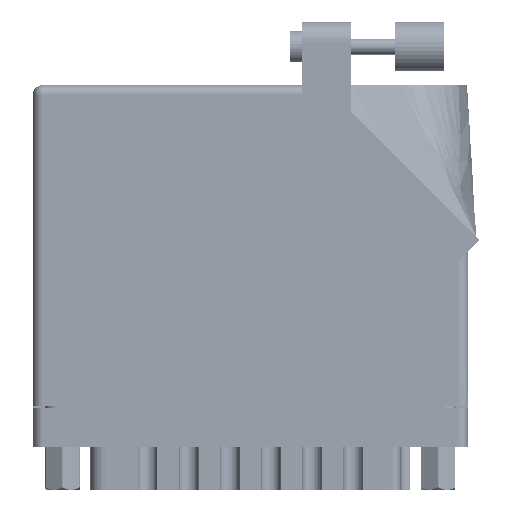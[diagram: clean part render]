
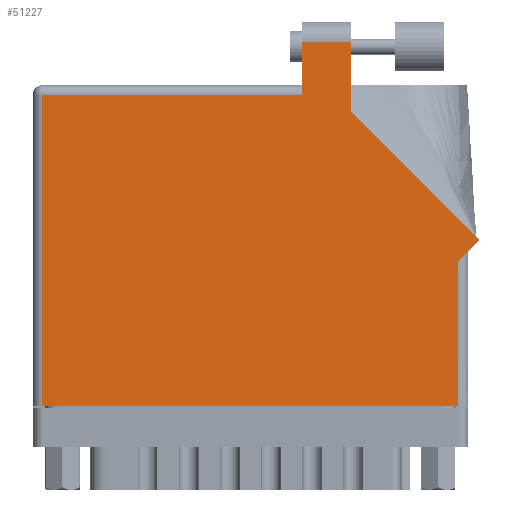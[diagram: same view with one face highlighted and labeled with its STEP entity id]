
A CAD part, front view. The second image highlights one B-rep face of the part: STEP entity #51227.
In plain terms, the highlighted face is planar.
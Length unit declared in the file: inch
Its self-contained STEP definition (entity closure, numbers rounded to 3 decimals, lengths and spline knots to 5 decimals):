
#69 = EDGE_CURVE ( 'NONE', #58738, #90624, #96330, .T. ) ;
#120 = VERTEX_POINT ( 'NONE', #54953 ) ;
#1323 = ORIENTED_EDGE ( 'NONE', *, *, #90444, .T. ) ;
#2523 = CARTESIAN_POINT ( 'NONE',  ( 0.062, 0., 0. ) ) ;
#3056 = ORIENTED_EDGE ( 'NONE', *, *, #69, .T. ) ;
#7707 = CARTESIAN_POINT ( 'NONE',  ( 2.755, 0.98, 0. ) ) ;
#7868 = DIRECTION ( 'NONE',  ( -0.707, 0.707, 0. ) ) ;
#9146 = LINE ( 'NONE', #7707, #66807 ) ;
#12510 = DIRECTION ( 'NONE',  ( 0., 0., -1. ) ) ;
#13361 = VECTOR ( 'NONE', #80149, 39.37008 ) ;
#14451 = CARTESIAN_POINT ( 'NONE',  ( 1.705, 1.968, 0. ) ) ;
#14509 = CARTESIAN_POINT ( 'NONE',  ( 0., 1.968, 0. ) ) ;
#16419 = LINE ( 'NONE', #42456, #101014 ) ;
#16767 = VECTOR ( 'NONE', #7868, 39.37008 ) ;
#20157 = LINE ( 'NONE', #26594, #27885 ) ;
#26452 = VERTEX_POINT ( 'NONE', #14451 ) ;
#26594 = CARTESIAN_POINT ( 'NONE',  ( 0.062, 0., 0. ) ) ;
#27885 = VECTOR ( 'NONE', #75751, 39.37008 ) ;
#28633 = LINE ( 'NONE', #75837, #69703 ) ;
#28959 = PLANE ( 'NONE',  #84256 ) ;
#30396 = EDGE_CURVE ( 'NONE', #26452, #61078, #36361, .T. ) ;
#31133 = CARTESIAN_POINT ( 'NONE',  ( 1.705, 2.305, 0. ) ) ;
#31562 = LINE ( 'NONE', #98910, #35449 ) ;
#32797 = CARTESIAN_POINT ( 'NONE',  ( 0.062, 1.968, 0. ) ) ;
#33068 = CARTESIAN_POINT ( 'NONE',  ( 1.705, 2.305, 0. ) ) ;
#35449 = VECTOR ( 'NONE', #82160, 39.37008 ) ;
#35515 = ORIENTED_EDGE ( 'NONE', *, *, #80331, .T. ) ;
#35644 = DIRECTION ( 'NONE',  ( 0., 1., 0. ) ) ;
#36361 = LINE ( 'NONE', #14509, #13361 ) ;
#36770 = VERTEX_POINT ( 'NONE', #53241 ) ;
#42456 = CARTESIAN_POINT ( 'NONE',  ( 2.012, 1.86442, 0. ) ) ;
#42857 = ORIENTED_EDGE ( 'NONE', *, *, #71810, .T. ) ;
#44968 = EDGE_CURVE ( 'NONE', #70366, #120, #48867, .T. ) ;
#48357 = ORIENTED_EDGE ( 'NONE', *, *, #69856, .T. ) ;
#48867 = LINE ( 'NONE', #105959, #16767 ) ;
#49530 = ORIENTED_EDGE ( 'NONE', *, *, #83313, .T. ) ;
#51227 = ADVANCED_FACE ( 'NONE', ( #67690 ), #28959, .F. ) ;
#53241 = CARTESIAN_POINT ( 'NONE',  ( 2.693, 0.918, 0. ) ) ;
#54953 = CARTESIAN_POINT ( 'NONE',  ( 2.012, 1.86442, 0. ) ) ;
#57809 = DIRECTION ( 'NONE',  ( 0.707, 0.707, 0. ) ) ;
#58738 = VERTEX_POINT ( 'NONE', #2523 ) ;
#61078 = VERTEX_POINT ( 'NONE', #32797 ) ;
#61192 = CARTESIAN_POINT ( 'NONE',  ( 0., 2.03, 0. ) ) ;
#61625 = EDGE_LOOP ( 'NONE', ( #1323, #42857, #49530, #95644, #48357, #3056, #98274, #35515, #93566 ) ) ;
#64730 = VERTEX_POINT ( 'NONE', #76283 ) ;
#66807 = VECTOR ( 'NONE', #57809, 39.37008 ) ;
#67690 = FACE_OUTER_BOUND ( 'NONE', #61625, .T. ) ;
#69703 = VECTOR ( 'NONE', #35644, 39.37008 ) ;
#69838 = LINE ( 'NONE', #31133, #72409 ) ;
#69856 = EDGE_CURVE ( 'NONE', #61078, #58738, #20157, .T. ) ;
#70366 = VERTEX_POINT ( 'NONE', #84223 ) ;
#71810 = EDGE_CURVE ( 'NONE', #64730, #95171, #69838, .T. ) ;
#72409 = VECTOR ( 'NONE', #88841, 39.37008 ) ;
#74559 = VECTOR ( 'NONE', #93304, 39.37008 ) ;
#75751 = DIRECTION ( 'NONE',  ( 0., -1., 0. ) ) ;
#75837 = CARTESIAN_POINT ( 'NONE',  ( 2.693, 0.98, 0. ) ) ;
#76283 = CARTESIAN_POINT ( 'NONE',  ( 2.012, 2.305, 0. ) ) ;
#80149 = DIRECTION ( 'NONE',  ( -1., 0., 0. ) ) ;
#80331 = EDGE_CURVE ( 'NONE', #36770, #70366, #9146, .T. ) ;
#82160 = DIRECTION ( 'NONE',  ( 0., -1., 0. ) ) ;
#83313 = EDGE_CURVE ( 'NONE', #95171, #26452, #31562, .T. ) ;
#84223 = CARTESIAN_POINT ( 'NONE',  ( 2.82571, 1.05071, 0. ) ) ;
#84256 = AXIS2_PLACEMENT_3D ( 'NONE', #61192, #12510, #103090 ) ;
#85108 = CARTESIAN_POINT ( 'NONE',  ( 0., 0., 0. ) ) ;
#86343 = EDGE_CURVE ( 'NONE', #90624, #36770, #28633, .T. ) ;
#88841 = DIRECTION ( 'NONE',  ( -1., 0., 0. ) ) ;
#90444 = EDGE_CURVE ( 'NONE', #120, #64730, #16419, .T. ) ;
#90624 = VERTEX_POINT ( 'NONE', #92630 ) ;
#92630 = CARTESIAN_POINT ( 'NONE',  ( 2.693, 0., 0. ) ) ;
#93304 = DIRECTION ( 'NONE',  ( 1., 0., 0. ) ) ;
#93566 = ORIENTED_EDGE ( 'NONE', *, *, #44968, .T. ) ;
#95171 = VERTEX_POINT ( 'NONE', #33068 ) ;
#95644 = ORIENTED_EDGE ( 'NONE', *, *, #30396, .T. ) ;
#96330 = LINE ( 'NONE', #85108, #74559 ) ;
#98274 = ORIENTED_EDGE ( 'NONE', *, *, #86343, .T. ) ;
#98910 = CARTESIAN_POINT ( 'NONE',  ( 1.705, 2.03, 0. ) ) ;
#99058 = DIRECTION ( 'NONE',  ( 0., 1., 0. ) ) ;
#101014 = VECTOR ( 'NONE', #99058, 39.37008 ) ;
#103090 = DIRECTION ( 'NONE',  ( -1., 0., 0. ) ) ;
#105959 = CARTESIAN_POINT ( 'NONE',  ( 2.82571, 1.05071, 0. ) ) ;
